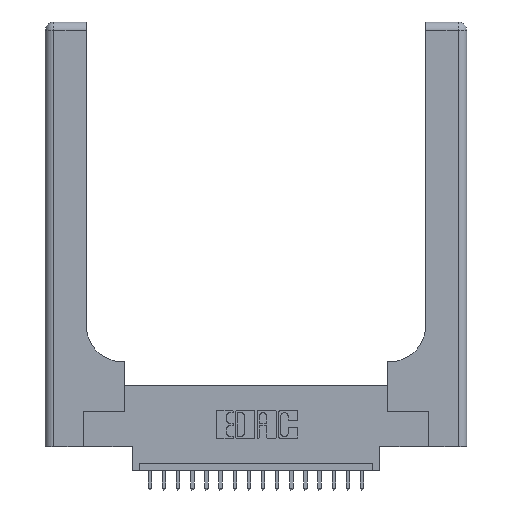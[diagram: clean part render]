
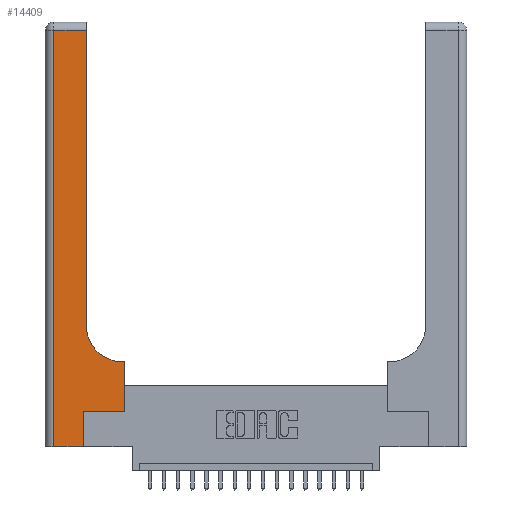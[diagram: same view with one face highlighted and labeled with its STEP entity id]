
A CAD part, top view. The second image highlights one B-rep face of the part: STEP entity #14409.
In plain terms, the highlighted planar face has unit normal (0, 0, 1).
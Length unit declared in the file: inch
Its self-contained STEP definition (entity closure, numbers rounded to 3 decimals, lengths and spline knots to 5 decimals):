
#163 = ORIENTED_EDGE ( 'NONE', *, *, #3297, .T. ) ;
#248 = VERTEX_POINT ( 'NONE', #12783 ) ;
#936 = VERTEX_POINT ( 'NONE', #12527 ) ;
#949 = VECTOR ( 'NONE', #2036, 39.37008 ) ;
#1041 = LINE ( 'NONE', #4192, #18408 ) ;
#1166 = ORIENTED_EDGE ( 'NONE', *, *, #20532, .T. ) ;
#1204 = CARTESIAN_POINT ( 'NONE',  ( 0.269, 0., 0.37 ) ) ;
#1479 = LINE ( 'NONE', #20730, #5756 ) ;
#2036 = DIRECTION ( 'NONE',  ( -1., 0., 0. ) ) ;
#2278 = VECTOR ( 'NONE', #3090, 39.37008 ) ;
#2641 = LINE ( 'NONE', #13968, #12752 ) ;
#2686 = DIRECTION ( 'NONE',  ( 0., 1., 0. ) ) ;
#2799 = CIRCLE ( 'NONE', #5791, 0.25 ) ;
#2859 = LINE ( 'NONE', #4436, #19508 ) ;
#3090 = DIRECTION ( 'NONE',  ( 0., 1., 0. ) ) ;
#3297 = EDGE_CURVE ( 'NONE', #12091, #12635, #7041, .T. ) ;
#3572 = DIRECTION ( 'NONE',  ( 0., 1., 0. ) ) ;
#4192 = CARTESIAN_POINT ( 'NONE',  ( 0.269, 0.25, 0.37 ) ) ;
#4310 = CARTESIAN_POINT ( 'NONE',  ( 0.2915, 0.85, 0.37 ) ) ;
#4436 = CARTESIAN_POINT ( 'NONE',  ( 0., 2.94, 0.37 ) ) ;
#4801 = ORIENTED_EDGE ( 'NONE', *, *, #10893, .T. ) ;
#5287 = VERTEX_POINT ( 'NONE', #4310 ) ;
#5419 = VECTOR ( 'NONE', #3572, 39.37008 ) ;
#5702 = ORIENTED_EDGE ( 'NONE', *, *, #7310, .T. ) ;
#5756 = VECTOR ( 'NONE', #19107, 39.37008 ) ;
#5791 = AXIS2_PLACEMENT_3D ( 'NONE', #13500, #16446, #18329 ) ;
#6170 = CARTESIAN_POINT ( 'NONE',  ( 0., 3., 0.37 ) ) ;
#6979 = CARTESIAN_POINT ( 'NONE',  ( 0.2915, 0.6, 0.37 ) ) ;
#7041 = LINE ( 'NONE', #18836, #18601 ) ;
#7310 = EDGE_CURVE ( 'NONE', #248, #5287, #2799, .T. ) ;
#7481 = AXIS2_PLACEMENT_3D ( 'NONE', #6170, #20559, #17325 ) ;
#7646 = FACE_OUTER_BOUND ( 'NONE', #19274, .T. ) ;
#7742 = CARTESIAN_POINT ( 'NONE',  ( 0.5585, 0.25, 0.37 ) ) ;
#8295 = EDGE_CURVE ( 'NONE', #14596, #9685, #19924, .T. ) ;
#8844 = EDGE_CURVE ( 'NONE', #10973, #14596, #1041, .T. ) ;
#9685 = VERTEX_POINT ( 'NONE', #11631 ) ;
#9736 = CARTESIAN_POINT ( 'NONE',  ( 0.5585, 0.25, 0.37 ) ) ;
#10893 = EDGE_CURVE ( 'NONE', #12635, #11829, #1479, .T. ) ;
#10973 = VERTEX_POINT ( 'NONE', #13118 ) ;
#11087 = PLANE ( 'NONE',  #7481 ) ;
#11454 = ORIENTED_EDGE ( 'NONE', *, *, #8295, .T. ) ;
#11631 = CARTESIAN_POINT ( 'NONE',  ( 0.5585, 0.6, 0.37 ) ) ;
#11777 = LINE ( 'NONE', #6979, #949 ) ;
#11829 = VERTEX_POINT ( 'NONE', #1204 ) ;
#12091 = VERTEX_POINT ( 'NONE', #19432 ) ;
#12209 = DIRECTION ( 'NONE',  ( 1., 0., 0. ) ) ;
#12527 = CARTESIAN_POINT ( 'NONE',  ( 0.2915, 2.94, 0.37 ) ) ;
#12635 = VERTEX_POINT ( 'NONE', #20824 ) ;
#12752 = VECTOR ( 'NONE', #2686, 39.37008 ) ;
#12783 = CARTESIAN_POINT ( 'NONE',  ( 0.5415, 0.6, 0.37 ) ) ;
#13118 = CARTESIAN_POINT ( 'NONE',  ( 0.269, 0.25, 0.37 ) ) ;
#13226 = CARTESIAN_POINT ( 'NONE',  ( 0.269, 0., 0.37 ) ) ;
#13454 = ORIENTED_EDGE ( 'NONE', *, *, #8844, .T. ) ;
#13500 = CARTESIAN_POINT ( 'NONE',  ( 0.5415, 0.85, 0.37 ) ) ;
#13968 = CARTESIAN_POINT ( 'NONE',  ( 0.2915, 3., 0.37 ) ) ;
#14409 = ADVANCED_FACE ( 'NONE', ( #7646 ), #11087, .F. ) ;
#14596 = VERTEX_POINT ( 'NONE', #9736 ) ;
#14713 = LINE ( 'NONE', #13226, #5419 ) ;
#15613 = EDGE_CURVE ( 'NONE', #5287, #936, #2641, .T. ) ;
#15696 = DIRECTION ( 'NONE',  ( -1., 0., 0. ) ) ;
#16244 = EDGE_CURVE ( 'NONE', #936, #12091, #2859, .T. ) ;
#16446 = DIRECTION ( 'NONE',  ( 0., 0., -1. ) ) ;
#16462 = EDGE_CURVE ( 'NONE', #11829, #10973, #14713, .T. ) ;
#17325 = DIRECTION ( 'NONE',  ( -1., 0., 0. ) ) ;
#17467 = ORIENTED_EDGE ( 'NONE', *, *, #16462, .T. ) ;
#18329 = DIRECTION ( 'NONE',  ( 1., 0., 0. ) ) ;
#18408 = VECTOR ( 'NONE', #12209, 39.37008 ) ;
#18601 = VECTOR ( 'NONE', #20239, 39.37008 ) ;
#18836 = CARTESIAN_POINT ( 'NONE',  ( 0.06, 3., 0.37 ) ) ;
#19107 = DIRECTION ( 'NONE',  ( 1., 0., 0. ) ) ;
#19274 = EDGE_LOOP ( 'NONE', ( #20464, #20254, #163, #4801, #17467, #13454, #11454, #1166, #5702 ) ) ;
#19432 = CARTESIAN_POINT ( 'NONE',  ( 0.06, 2.94, 0.37 ) ) ;
#19508 = VECTOR ( 'NONE', #15696, 39.37008 ) ;
#19924 = LINE ( 'NONE', #7742, #2278 ) ;
#20239 = DIRECTION ( 'NONE',  ( 0., -1., 0. ) ) ;
#20254 = ORIENTED_EDGE ( 'NONE', *, *, #16244, .T. ) ;
#20464 = ORIENTED_EDGE ( 'NONE', *, *, #15613, .T. ) ;
#20532 = EDGE_CURVE ( 'NONE', #9685, #248, #11777, .T. ) ;
#20559 = DIRECTION ( 'NONE',  ( 0., 0., -1. ) ) ;
#20730 = CARTESIAN_POINT ( 'NONE',  ( 0., 0., 0.37 ) ) ;
#20824 = CARTESIAN_POINT ( 'NONE',  ( 0.06, 0., 0.37 ) ) ;
